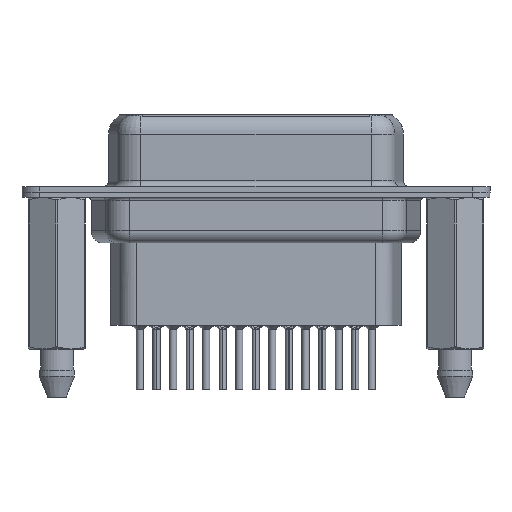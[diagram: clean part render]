
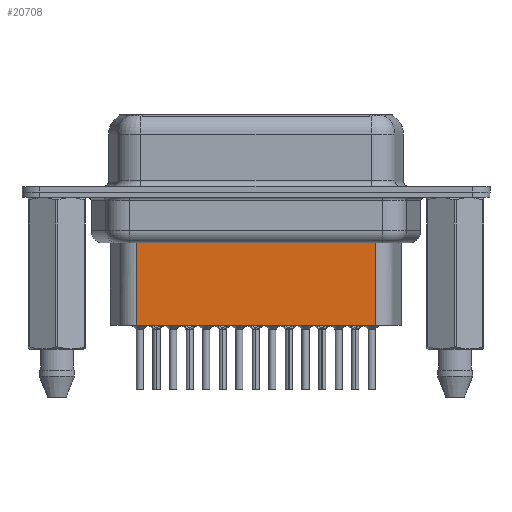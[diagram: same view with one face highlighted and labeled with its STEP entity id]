
A CAD part, front view. The second image highlights one B-rep face of the part: STEP entity #20708.
In plain terms, the highlighted planar face has unit normal (0, -1, 0).
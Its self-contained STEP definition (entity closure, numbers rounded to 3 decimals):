
#85 = VERTEX_POINT ( 'NONE', #831 ) ;
#615 = CARTESIAN_POINT ( 'NONE',  ( 6.681, -3.5, -3.1 ) ) ;
#831 = CARTESIAN_POINT ( 'NONE',  ( 26.619, -3.5, -11.15 ) ) ;
#2086 = VECTOR ( 'NONE', #16301, 1000. ) ;
#4105 = LINE ( 'NONE', #23432, #20867 ) ;
#4427 = PLANE ( 'NONE',  #7643 ) ;
#4913 = DIRECTION ( 'NONE',  ( 1., 0., 0. ) ) ;
#5113 = ORIENTED_EDGE ( 'NONE', *, *, #7816, .F. ) ;
#5284 = CARTESIAN_POINT ( 'NONE',  ( 6.681, -3.5, -11.15 ) ) ;
#5471 = VECTOR ( 'NONE', #21670, 1000. ) ;
#5869 = VERTEX_POINT ( 'NONE', #5284 ) ;
#5994 = DIRECTION ( 'NONE',  ( 0., 0., -1. ) ) ;
#6447 = DIRECTION ( 'NONE',  ( 0., -1., 0. ) ) ;
#6495 = LINE ( 'NONE', #16683, #2086 ) ;
#7436 = VERTEX_POINT ( 'NONE', #8580 ) ;
#7643 = AXIS2_PLACEMENT_3D ( 'NONE', #615, #6447, #4913 ) ;
#7816 = EDGE_CURVE ( 'NONE', #85, #5869, #6495, .T. ) ;
#8045 = LINE ( 'NONE', #23799, #5471 ) ;
#8580 = CARTESIAN_POINT ( 'NONE',  ( 6.681, -3.5, -4.097 ) ) ;
#8682 = ORIENTED_EDGE ( 'NONE', *, *, #8986, .F. ) ;
#8986 = EDGE_CURVE ( 'NONE', #14701, #85, #4105, .T. ) ;
#10536 = EDGE_CURVE ( 'NONE', #7436, #5869, #8045, .T. ) ;
#10780 = EDGE_CURVE ( 'NONE', #14701, #7436, #16920, .T. ) ;
#10928 = CARTESIAN_POINT ( 'NONE',  ( 26.619, -3.5, -4.097 ) ) ;
#13112 = CARTESIAN_POINT ( 'NONE',  ( 6.434, -3.5, -4.097 ) ) ;
#14701 = VERTEX_POINT ( 'NONE', #10928 ) ;
#14952 = EDGE_LOOP ( 'NONE', ( #8682, #16524, #21375, #5113 ) ) ;
#15885 = FACE_OUTER_BOUND ( 'NONE', #14952, .T. ) ;
#16301 = DIRECTION ( 'NONE',  ( -1., 0., 0. ) ) ;
#16524 = ORIENTED_EDGE ( 'NONE', *, *, #10780, .T. ) ;
#16683 = CARTESIAN_POINT ( 'NONE',  ( 6.681, -3.5, -11.15 ) ) ;
#16920 = LINE ( 'NONE', #13112, #17782 ) ;
#17782 = VECTOR ( 'NONE', #18708, 1000. ) ;
#18708 = DIRECTION ( 'NONE',  ( -1., 0., 0. ) ) ;
#20708 = ADVANCED_FACE ( 'NONE', ( #15885 ), #4427, .T. ) ;
#20867 = VECTOR ( 'NONE', #5994, 1000. ) ;
#21375 = ORIENTED_EDGE ( 'NONE', *, *, #10536, .T. ) ;
#21670 = DIRECTION ( 'NONE',  ( 0., 0., -1. ) ) ;
#23432 = CARTESIAN_POINT ( 'NONE',  ( 26.619, -3.5, -3.1 ) ) ;
#23799 = CARTESIAN_POINT ( 'NONE',  ( 6.681, -3.5, -3.1 ) ) ;
